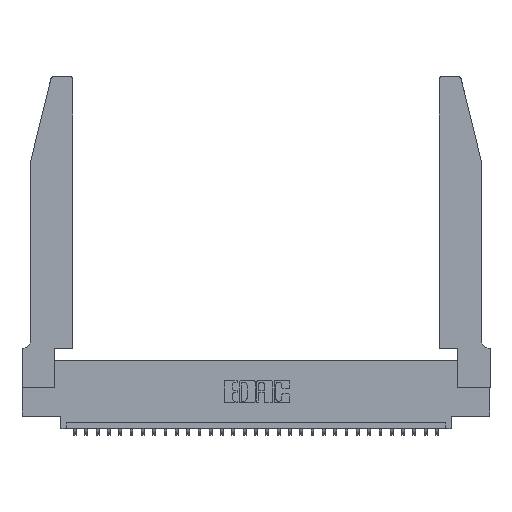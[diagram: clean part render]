
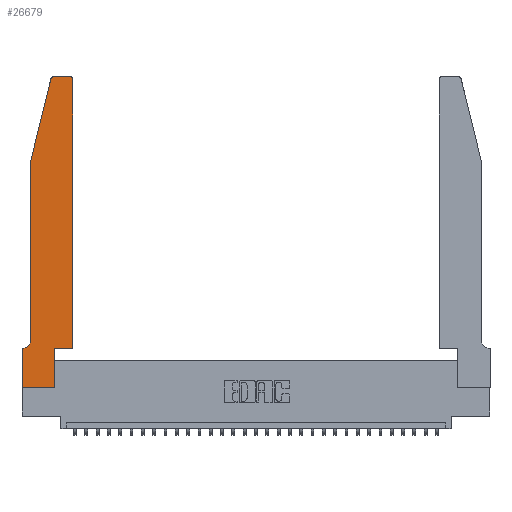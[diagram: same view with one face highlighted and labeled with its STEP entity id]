
A CAD part, top view. The second image highlights one B-rep face of the part: STEP entity #26679.
In plain terms, the highlighted planar face has unit normal (0, 0, 1).
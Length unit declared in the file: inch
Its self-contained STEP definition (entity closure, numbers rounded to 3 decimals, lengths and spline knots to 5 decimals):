
#207 = LINE ( 'NONE', #28040, #23405 ) ;
#269 = DIRECTION ( 'NONE',  ( 0., 0., 1. ) ) ;
#318 = CARTESIAN_POINT ( 'NONE',  ( 0.25487, 2.72718, 0.37 ) ) ;
#549 = LINE ( 'NONE', #27831, #26746 ) ;
#791 = CARTESIAN_POINT ( 'NONE',  ( 0.0055, 0.35, 0.37 ) ) ;
#837 = ORIENTED_EDGE ( 'NONE', *, *, #16456, .T. ) ;
#1123 = ORIENTED_EDGE ( 'NONE', *, *, #16081, .T. ) ;
#1150 = CARTESIAN_POINT ( 'NONE',  ( 0.2865, 0.35, 0.37 ) ) ;
#1190 = EDGE_CURVE ( 'NONE', #13675, #15238, #549, .T. ) ;
#1571 = EDGE_LOOP ( 'NONE', ( #31006, #21788, #13504, #27742, #26148, #15095, #14405, #30617, #837, #14849, #27445, #1123 ) ) ;
#1699 = DIRECTION ( 'NONE',  ( 1., 0., 0. ) ) ;
#3556 = DIRECTION ( 'NONE',  ( 0., -1., 0. ) ) ;
#3689 = DIRECTION ( 'NONE',  ( -0.239, -0.971, 0. ) ) ;
#3736 = CARTESIAN_POINT ( 'NONE',  ( 0.4205, 2.75, 0.37 ) ) ;
#3803 = CARTESIAN_POINT ( 'NONE',  ( 0., 0., 0.37 ) ) ;
#5160 = FACE_OUTER_BOUND ( 'NONE', #1571, .T. ) ;
#5342 = LINE ( 'NONE', #17802, #7219 ) ;
#6003 = LINE ( 'NONE', #29222, #10829 ) ;
#6465 = CARTESIAN_POINT ( 'NONE',  ( 0., 0.35, 0.37 ) ) ;
#6913 = DIRECTION ( 'NONE',  ( 0., 0., 1. ) ) ;
#7108 = VERTEX_POINT ( 'NONE', #18497 ) ;
#7219 = VECTOR ( 'NONE', #3556, 39.37008 ) ;
#7461 = CARTESIAN_POINT ( 'NONE',  ( 0., 0., 0.37 ) ) ;
#7653 = LINE ( 'NONE', #24347, #12125 ) ;
#7904 = CARTESIAN_POINT ( 'NONE',  ( 0.284, 2.75, 0.37 ) ) ;
#8116 = DIRECTION ( 'NONE',  ( -1., 0., 0. ) ) ;
#8856 = CARTESIAN_POINT ( 'NONE',  ( 0.2865, 0., 0.37 ) ) ;
#9041 = VERTEX_POINT ( 'NONE', #791 ) ;
#9276 = EDGE_CURVE ( 'NONE', #14178, #23951, #13950, .T. ) ;
#9278 = CARTESIAN_POINT ( 'NONE',  ( 0.284, 2.72, 0.37 ) ) ;
#9860 = CARTESIAN_POINT ( 'NONE',  ( 0.4505, 2.72, 0.37 ) ) ;
#9889 = VECTOR ( 'NONE', #29424, 39.37008 ) ;
#10003 = DIRECTION ( 'NONE',  ( -1., 0., 0. ) ) ;
#10459 = EDGE_CURVE ( 'NONE', #15238, #20939, #5342, .T. ) ;
#10829 = VECTOR ( 'NONE', #14555, 39.37008 ) ;
#10884 = VERTEX_POINT ( 'NONE', #7904 ) ;
#11886 = EDGE_CURVE ( 'NONE', #20939, #9041, #29528, .T. ) ;
#12125 = VECTOR ( 'NONE', #10003, 39.37008 ) ;
#12215 = VERTEX_POINT ( 'NONE', #8856 ) ;
#12601 = EDGE_CURVE ( 'NONE', #18313, #26316, #22407, .T. ) ;
#12651 = CIRCLE ( 'NONE', #21871, 0.03 ) ;
#13504 = ORIENTED_EDGE ( 'NONE', *, *, #1190, .T. ) ;
#13675 = VERTEX_POINT ( 'NONE', #318 ) ;
#13950 = LINE ( 'NONE', #27542, #9889 ) ;
#14178 = VERTEX_POINT ( 'NONE', #14803 ) ;
#14405 = ORIENTED_EDGE ( 'NONE', *, *, #12601, .T. ) ;
#14555 = DIRECTION ( 'NONE',  ( 1., 0., 0. ) ) ;
#14672 = LINE ( 'NONE', #26922, #25996 ) ;
#14803 = CARTESIAN_POINT ( 'NONE',  ( 0.4505, 0.35, 0.37 ) ) ;
#14849 = ORIENTED_EDGE ( 'NONE', *, *, #28490, .T. ) ;
#14946 = CIRCLE ( 'NONE', #24254, 0.03 ) ;
#15095 = ORIENTED_EDGE ( 'NONE', *, *, #22874, .T. ) ;
#15238 = VERTEX_POINT ( 'NONE', #17761 ) ;
#16081 = EDGE_CURVE ( 'NONE', #23951, #30919, #14946, .T. ) ;
#16086 = AXIS2_PLACEMENT_3D ( 'NONE', #29444, #22136, #8116 ) ;
#16175 = PLANE ( 'NONE',  #21914 ) ;
#16276 = CARTESIAN_POINT ( 'NONE',  ( 0.4205, 2.72, 0.37 ) ) ;
#16383 = DIRECTION ( 'NONE',  ( 1., 0., 0. ) ) ;
#16456 = EDGE_CURVE ( 'NONE', #12215, #7108, #17567, .T. ) ;
#16495 = DIRECTION ( 'NONE',  ( 1., 0., 0. ) ) ;
#17074 = CARTESIAN_POINT ( 'NONE',  ( 0.0755, 0.42, 0.37 ) ) ;
#17567 = LINE ( 'NONE', #1150, #19071 ) ;
#17761 = CARTESIAN_POINT ( 'NONE',  ( 0.0755, 2., 0.37 ) ) ;
#17802 = CARTESIAN_POINT ( 'NONE',  ( 0.0755, 2., 0.37 ) ) ;
#17887 = VECTOR ( 'NONE', #27388, 39.37008 ) ;
#18006 = EDGE_CURVE ( 'NONE', #10884, #13675, #12651, .T. ) ;
#18313 = VERTEX_POINT ( 'NONE', #6465 ) ;
#18497 = CARTESIAN_POINT ( 'NONE',  ( 0.2865, 0.35, 0.37 ) ) ;
#18792 = CARTESIAN_POINT ( 'NONE',  ( 0., 0.35, 0.37 ) ) ;
#19071 = VECTOR ( 'NONE', #20354, 39.37008 ) ;
#20354 = DIRECTION ( 'NONE',  ( 0., 1., 0. ) ) ;
#20543 = EDGE_CURVE ( 'NONE', #30919, #10884, #7653, .T. ) ;
#20939 = VERTEX_POINT ( 'NONE', #17074 ) ;
#21788 = ORIENTED_EDGE ( 'NONE', *, *, #18006, .T. ) ;
#21871 = AXIS2_PLACEMENT_3D ( 'NONE', #9278, #269, #16495 ) ;
#21914 = AXIS2_PLACEMENT_3D ( 'NONE', #18792, #25981, #16383 ) ;
#22136 = DIRECTION ( 'NONE',  ( 0., 0., -1. ) ) ;
#22407 = LINE ( 'NONE', #3803, #17887 ) ;
#22413 = DIRECTION ( 'NONE',  ( -1., 0., 0. ) ) ;
#22874 = EDGE_CURVE ( 'NONE', #9041, #18313, #14672, .T. ) ;
#23405 = VECTOR ( 'NONE', #30467, 39.37008 ) ;
#23951 = VERTEX_POINT ( 'NONE', #9860 ) ;
#24254 = AXIS2_PLACEMENT_3D ( 'NONE', #16276, #6913, #1699 ) ;
#24347 = CARTESIAN_POINT ( 'NONE',  ( 0.2605, 2.75, 0.37 ) ) ;
#25113 = EDGE_CURVE ( 'NONE', #26316, #12215, #6003, .T. ) ;
#25981 = DIRECTION ( 'NONE',  ( 0., 0., 1. ) ) ;
#25996 = VECTOR ( 'NONE', #22413, 39.37008 ) ;
#26148 = ORIENTED_EDGE ( 'NONE', *, *, #11886, .T. ) ;
#26316 = VERTEX_POINT ( 'NONE', #7461 ) ;
#26679 = ADVANCED_FACE ( 'NONE', ( #5160 ), #16175, .T. ) ;
#26746 = VECTOR ( 'NONE', #3689, 39.37008 ) ;
#26922 = CARTESIAN_POINT ( 'NONE',  ( 0.0755, 0.35, 0.37 ) ) ;
#27388 = DIRECTION ( 'NONE',  ( 0., -1., 0. ) ) ;
#27445 = ORIENTED_EDGE ( 'NONE', *, *, #9276, .T. ) ;
#27542 = CARTESIAN_POINT ( 'NONE',  ( 0.4505, 0.35, 0.37 ) ) ;
#27742 = ORIENTED_EDGE ( 'NONE', *, *, #10459, .T. ) ;
#27831 = CARTESIAN_POINT ( 'NONE',  ( 0.0755, 2., 0.37 ) ) ;
#28040 = CARTESIAN_POINT ( 'NONE',  ( 0.4505, 0.35, 0.37 ) ) ;
#28490 = EDGE_CURVE ( 'NONE', #7108, #14178, #207, .T. ) ;
#29222 = CARTESIAN_POINT ( 'NONE',  ( 0., 0., 0.37 ) ) ;
#29424 = DIRECTION ( 'NONE',  ( 0., 1., 0. ) ) ;
#29444 = CARTESIAN_POINT ( 'NONE',  ( 0.0055, 0.42, 0.37 ) ) ;
#29528 = CIRCLE ( 'NONE', #16086, 0.07 ) ;
#30467 = DIRECTION ( 'NONE',  ( 1., 0., 0. ) ) ;
#30617 = ORIENTED_EDGE ( 'NONE', *, *, #25113, .T. ) ;
#30919 = VERTEX_POINT ( 'NONE', #3736 ) ;
#31006 = ORIENTED_EDGE ( 'NONE', *, *, #20543, .T. ) ;
